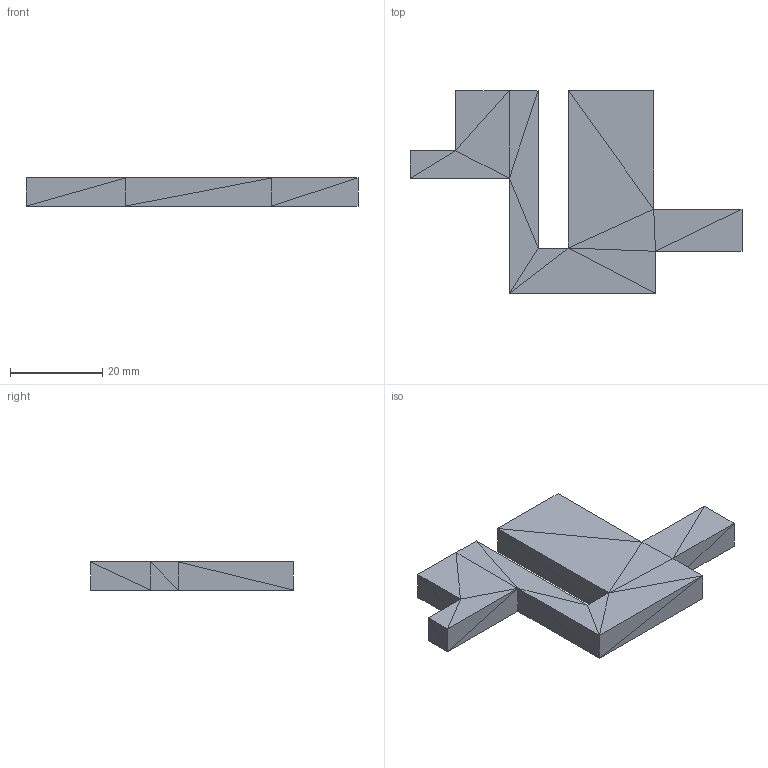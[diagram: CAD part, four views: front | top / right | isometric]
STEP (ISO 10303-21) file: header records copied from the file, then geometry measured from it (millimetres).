
FILE_DESCRIPTION(('FreeCAD Model'),'2;1');
FILE_NAME('Open CASCADE Shape Model','2021-09-30T12:00:38',('Author'),( ''),'Open CASCADE STEP processor 7.4','FreeCAD','Unknown');
FILE_SCHEMA(('AUTOMOTIVE_DESIGN { 1 0 10303 214 1 1 1 1 }'));
Length unit declared in the file: millimetre
Products named in the file (1): Trigger_Middle001_(Solid)
Bounding box: 72.14 x 44.07 x 6.1 mm (x, y, z)
Volume: 9860.3 mm3; surface area: 5068.3 mm2
Topology: 1 solids, 1 shells, 68 faces, 102 edges, 36 vertices
Faces by surface type: plane 68
Entity records: 2584 total; most frequent: CARTESIAN_POINT 513, DIRECTION 342, ORIENTED_EDGE 204, LINE 204, VECTOR 204, PCURVE 204, DEFINITIONAL_REPRESENTATION 204, EDGE_CURVE 102
